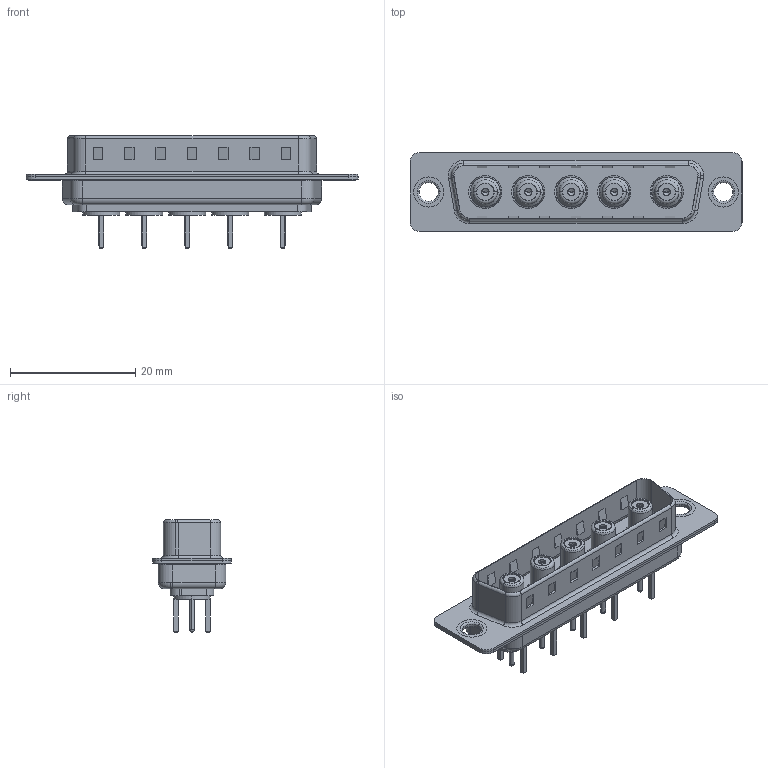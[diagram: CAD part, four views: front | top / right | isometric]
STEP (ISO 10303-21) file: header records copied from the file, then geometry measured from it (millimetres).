
FILE_DESCRIPTION (( 'STEP AP203' ), '1' );
FILE_NAME ('627-5W5-624-5T1.STEP', '2019-05-26T02:01:00', ( '' ), ( '' ), 'SwSTEP 2.0', 'SolidWorks 2016', '' );
FILE_SCHEMA (( 'CONFIG_CONTROL_DESIGN' ));
Length unit declared in the file: millimetre
Products named in the file (11): Locking Collar; Socket_Str; 627Combo Housing_5W5; Co-Ax Jack Assy_S; 627Combo Shell Rear_25 Contacts; 627-5W5-624-5T1; 627Combo Shell Front_25 Contacts; 627Combo Thru Hole Rivet; Co-Ax Jack_Straight PC Tail; Insulator Socket; Insulator Socket 2
Assembly tree (15 placements, depth 3):
  627-5W5-624-5T1
    627Combo Housing_5W5
    627Combo Shell Rear_25 Contacts
    627Combo Shell Front_25 Contacts
    627Combo Thru Hole Rivet  x2
    Co-Ax Jack Assy_S  x5
      Co-Ax Jack_Straight PC Tail
      Insulator Socket
      Insulator Socket 2
      Locking Collar
      Socket_Str
Bounding box: 53 x 12.6 x 17.9 mm (x, y, z)
Volume: 2748.5 mm3; surface area: 8548 mm2
Topology: 30 solids, 30 shells, 905 faces, 2120 edges, 1326 vertices
Faces by surface type: plane 406, cylinder 356, torus 78, cone 45, bspline 10, sphere 10
Entity records: 15072 total; most frequent: DIRECTION 2500, CARTESIAN_POINT 2464, ORIENTED_EDGE 2252, EDGE_CURVE 1126, AXIS2_PLACEMENT_3D 923, VERTEX_POINT 710, LINE 654, VECTOR 654
